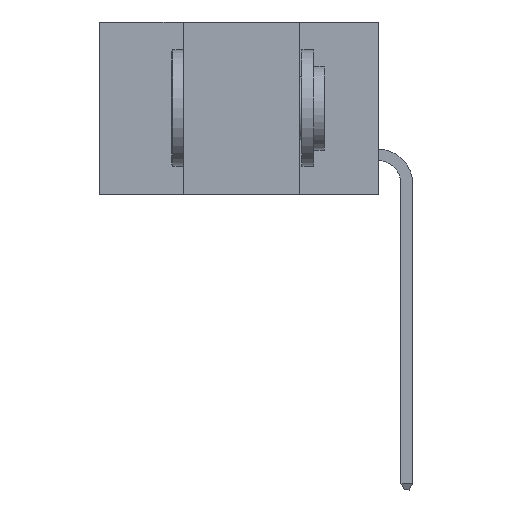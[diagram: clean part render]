
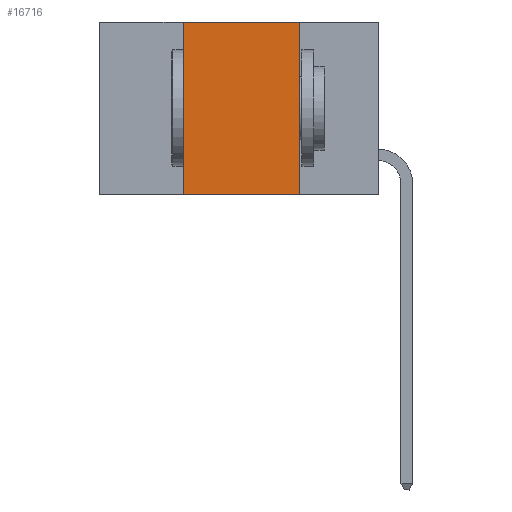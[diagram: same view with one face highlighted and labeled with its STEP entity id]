
A CAD part, left-side view. The second image highlights one B-rep face of the part: STEP entity #16716.
In plain terms, the highlighted planar face has unit normal (-1, 0, 0).
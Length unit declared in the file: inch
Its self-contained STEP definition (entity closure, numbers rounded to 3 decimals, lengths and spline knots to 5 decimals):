
#760 = CARTESIAN_POINT ( 'NONE',  ( 0., 0.6, -0.37 ) ) ;
#1049 = CARTESIAN_POINT ( 'NONE',  ( 0., 0.17, -0.37 ) ) ;
#1218 = ORIENTED_EDGE ( 'NONE', *, *, #10247, .F. ) ;
#2101 = VERTEX_POINT ( 'NONE', #3628 ) ;
#2572 = DIRECTION ( 'NONE',  ( 0., 0., -1. ) ) ;
#2758 = DIRECTION ( 'NONE',  ( 1., 0., 0. ) ) ;
#2974 = CARTESIAN_POINT ( 'NONE',  ( 0., 0.42, -0.37 ) ) ;
#3458 = ORIENTED_EDGE ( 'NONE', *, *, #19106, .T. ) ;
#3628 = CARTESIAN_POINT ( 'NONE',  ( 0., 0.42, 0. ) ) ;
#3832 = LINE ( 'NONE', #5470, #8167 ) ;
#4415 = FACE_OUTER_BOUND ( 'NONE', #7422, .T. ) ;
#5470 = CARTESIAN_POINT ( 'NONE',  ( 0., 0.6, 0. ) ) ;
#5487 = VERTEX_POINT ( 'NONE', #14494 ) ;
#5866 = AXIS2_PLACEMENT_3D ( 'NONE', #13120, #2758, #2572 ) ;
#5900 = DIRECTION ( 'NONE',  ( 0., 0., 1. ) ) ;
#6423 = DIRECTION ( 'NONE',  ( 0., -1., 0. ) ) ;
#7422 = EDGE_LOOP ( 'NONE', ( #1218, #10307, #9457, #3458 ) ) ;
#8167 = VECTOR ( 'NONE', #14274, 39.37008 ) ;
#8820 = VERTEX_POINT ( 'NONE', #1049 ) ;
#9200 = VERTEX_POINT ( 'NONE', #10011 ) ;
#9341 = EDGE_CURVE ( 'NONE', #5487, #2101, #15201, .T. ) ;
#9457 = ORIENTED_EDGE ( 'NONE', *, *, #9341, .F. ) ;
#10011 = CARTESIAN_POINT ( 'NONE',  ( 0., 0.17, 0. ) ) ;
#10124 = EDGE_CURVE ( 'NONE', #2101, #9200, #3832, .T. ) ;
#10247 = EDGE_CURVE ( 'NONE', #9200, #8820, #14660, .T. ) ;
#10307 = ORIENTED_EDGE ( 'NONE', *, *, #10124, .F. ) ;
#11323 = VECTOR ( 'NONE', #5900, 39.37008 ) ;
#13120 = CARTESIAN_POINT ( 'NONE',  ( 0., 0.6, 0. ) ) ;
#14274 = DIRECTION ( 'NONE',  ( 0., -1., 0. ) ) ;
#14494 = CARTESIAN_POINT ( 'NONE',  ( 0., 0.42, -0.37 ) ) ;
#14660 = LINE ( 'NONE', #18672, #18161 ) ;
#15201 = LINE ( 'NONE', #2974, #11323 ) ;
#15822 = LINE ( 'NONE', #760, #16553 ) ;
#16347 = PLANE ( 'NONE',  #5866 ) ;
#16553 = VECTOR ( 'NONE', #6423, 39.37008 ) ;
#16716 = ADVANCED_FACE ( 'NONE', ( #4415 ), #16347, .F. ) ;
#17221 = DIRECTION ( 'NONE',  ( 0., 0., -1. ) ) ;
#18161 = VECTOR ( 'NONE', #17221, 39.37008 ) ;
#18672 = CARTESIAN_POINT ( 'NONE',  ( 0., 0.17, -0.37 ) ) ;
#19106 = EDGE_CURVE ( 'NONE', #5487, #8820, #15822, .T. ) ;
